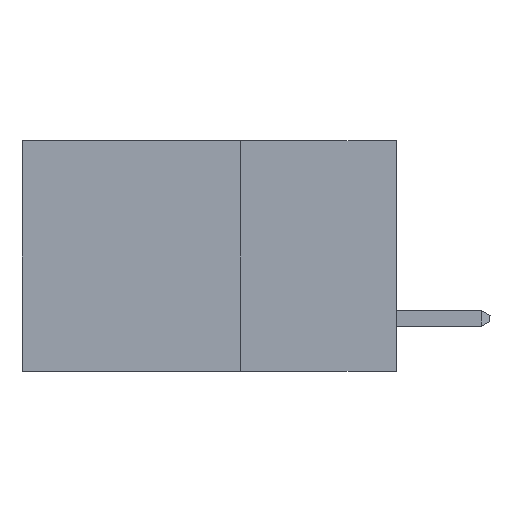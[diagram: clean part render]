
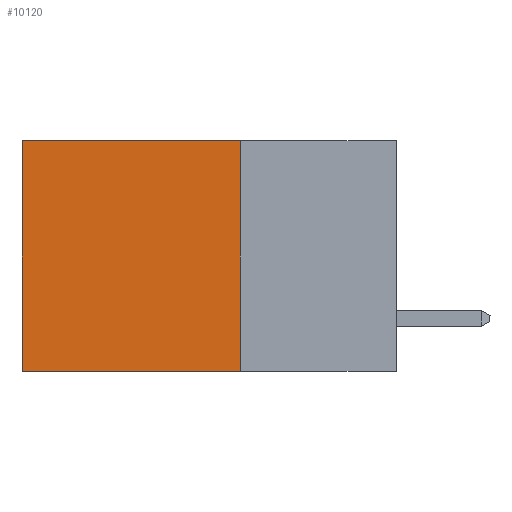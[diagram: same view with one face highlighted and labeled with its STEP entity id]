
A CAD part, left-side view. The second image highlights one B-rep face of the part: STEP entity #10120.
In plain terms, the highlighted planar face has unit normal (-1, 0, 0).
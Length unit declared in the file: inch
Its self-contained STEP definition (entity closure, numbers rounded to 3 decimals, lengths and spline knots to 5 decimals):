
#520 = LINE ( 'NONE', #3931, #9783 ) ;
#1143 = VERTEX_POINT ( 'NONE', #10980 ) ;
#1306 = VERTEX_POINT ( 'NONE', #3940 ) ;
#1403 = DIRECTION ( 'NONE',  ( 0., 0., -1. ) ) ;
#1821 = PLANE ( 'NONE',  #11273 ) ;
#2096 = LINE ( 'NONE', #11754, #3977 ) ;
#2565 = VECTOR ( 'NONE', #9263, 39.37008 ) ;
#3149 = ORIENTED_EDGE ( 'NONE', *, *, #9781, .T. ) ;
#3694 = DIRECTION ( 'NONE',  ( 1., 0., 0. ) ) ;
#3800 = EDGE_CURVE ( 'NONE', #1143, #7003, #520, .T. ) ;
#3931 = CARTESIAN_POINT ( 'NONE',  ( 0.2615, 0.25, -0.37 ) ) ;
#3940 = CARTESIAN_POINT ( 'NONE',  ( 0.2615, 0.6, 0. ) ) ;
#3977 = VECTOR ( 'NONE', #9978, 39.37008 ) ;
#4577 = LINE ( 'NONE', #6021, #6733 ) ;
#4629 = CARTESIAN_POINT ( 'NONE',  ( 0.2615, 0.25, -0.37 ) ) ;
#4709 = CARTESIAN_POINT ( 'NONE',  ( 0.2615, 0.25, -0.37 ) ) ;
#4872 = EDGE_CURVE ( 'NONE', #1143, #1306, #2096, .T. ) ;
#5287 = LINE ( 'NONE', #4709, #2565 ) ;
#5810 = DIRECTION ( 'NONE',  ( 0., 0., -1. ) ) ;
#6021 = CARTESIAN_POINT ( 'NONE',  ( 0.2615, 0.6, -0.37 ) ) ;
#6155 = ORIENTED_EDGE ( 'NONE', *, *, #4872, .T. ) ;
#6733 = VECTOR ( 'NONE', #1403, 39.37008 ) ;
#7003 = VERTEX_POINT ( 'NONE', #4629 ) ;
#8148 = VERTEX_POINT ( 'NONE', #8323 ) ;
#8247 = CARTESIAN_POINT ( 'NONE',  ( 0.2615, 0.25, -0.37 ) ) ;
#8296 = ORIENTED_EDGE ( 'NONE', *, *, #3800, .F. ) ;
#8323 = CARTESIAN_POINT ( 'NONE',  ( 0.2615, 0.6, -0.37 ) ) ;
#9263 = DIRECTION ( 'NONE',  ( 0., 1., 0. ) ) ;
#9505 = EDGE_CURVE ( 'NONE', #7003, #8148, #5287, .T. ) ;
#9781 = EDGE_CURVE ( 'NONE', #1306, #8148, #4577, .T. ) ;
#9783 = VECTOR ( 'NONE', #5810, 39.37008 ) ;
#9836 = EDGE_LOOP ( 'NONE', ( #3149, #10415, #8296, #6155 ) ) ;
#9978 = DIRECTION ( 'NONE',  ( 0., 1., 0. ) ) ;
#10072 = DIRECTION ( 'NONE',  ( 0., 0., -1. ) ) ;
#10120 = ADVANCED_FACE ( 'NONE', ( #11099 ), #1821, .F. ) ;
#10415 = ORIENTED_EDGE ( 'NONE', *, *, #9505, .F. ) ;
#10980 = CARTESIAN_POINT ( 'NONE',  ( 0.2615, 0.25, 0. ) ) ;
#11099 = FACE_OUTER_BOUND ( 'NONE', #9836, .T. ) ;
#11273 = AXIS2_PLACEMENT_3D ( 'NONE', #8247, #3694, #10072 ) ;
#11754 = CARTESIAN_POINT ( 'NONE',  ( 0.2615, 0.25, 0. ) ) ;
